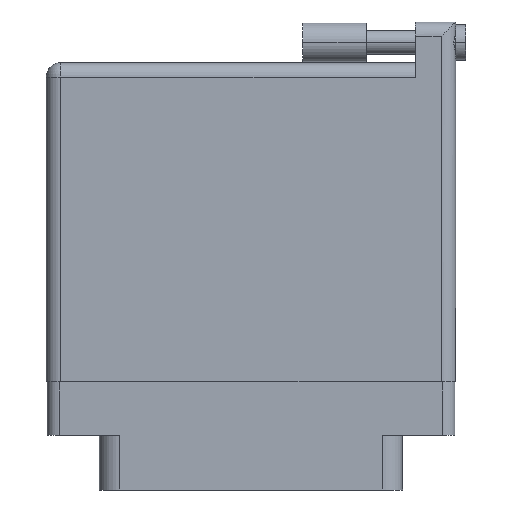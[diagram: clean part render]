
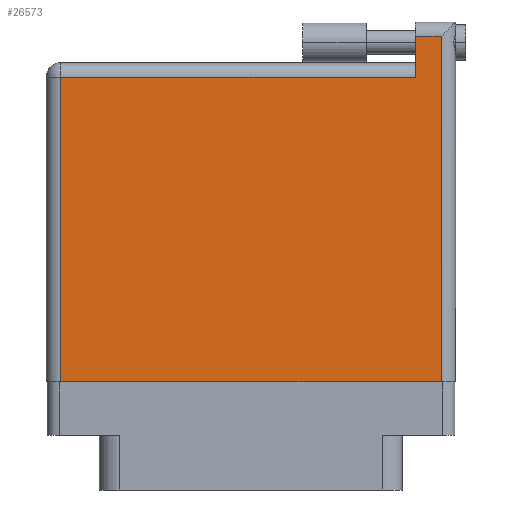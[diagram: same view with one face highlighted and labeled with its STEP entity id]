
A CAD part, front view. The second image highlights one B-rep face of the part: STEP entity #26573.
In plain terms, the highlighted face is planar.
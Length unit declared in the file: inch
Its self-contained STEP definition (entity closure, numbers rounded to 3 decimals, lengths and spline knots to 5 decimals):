
#132 = CARTESIAN_POINT ( 'NONE',  ( 1.938, 0., 0. ) ) ;
#151 = EDGE_CURVE ( 'NONE', #28569, #36948, #36484, .T. ) ;
#687 = LINE ( 'NONE', #1060, #37702 ) ;
#731 = EDGE_CURVE ( 'NONE', #36948, #12872, #7564, .T. ) ;
#1060 = CARTESIAN_POINT ( 'NONE',  ( 1.938, 1.766, 0. ) ) ;
#1543 = ORIENTED_EDGE ( 'NONE', *, *, #731, .T. ) ;
#2525 = EDGE_CURVE ( 'NONE', #10656, #7990, #35919, .T. ) ;
#2567 = DIRECTION ( 'NONE',  ( 1., 0., 0. ) ) ;
#6646 = EDGE_LOOP ( 'NONE', ( #20522, #17226, #30401, #1543, #36429, #10999 ) ) ;
#7318 = FACE_OUTER_BOUND ( 'NONE', #6646, .T. ) ;
#7564 = LINE ( 'NONE', #14222, #23853 ) ;
#7990 = VERTEX_POINT ( 'NONE', #132 ) ;
#8092 = EDGE_CURVE ( 'NONE', #7990, #28569, #687, .T. ) ;
#8253 = VERTEX_POINT ( 'NONE', #28527 ) ;
#10656 = VERTEX_POINT ( 'NONE', #20781 ) ;
#10724 = DIRECTION ( 'NONE',  ( 0., -1., 0. ) ) ;
#10999 = ORIENTED_EDGE ( 'NONE', *, *, #38059, .T. ) ;
#11106 = LINE ( 'NONE', #13863, #38313 ) ;
#12872 = VERTEX_POINT ( 'NONE', #20496 ) ;
#13474 = CARTESIAN_POINT ( 'NONE',  ( 0., 1.496, 0. ) ) ;
#13863 = CARTESIAN_POINT ( 'NONE',  ( 0.07, 0., 0. ) ) ;
#14222 = CARTESIAN_POINT ( 'NONE',  ( 1.811, 1.766, 0. ) ) ;
#14727 = DIRECTION ( 'NONE',  ( -1., 0., 0. ) ) ;
#17097 = VECTOR ( 'NONE', #2567, 39.37008 ) ;
#17226 = ORIENTED_EDGE ( 'NONE', *, *, #8092, .T. ) ;
#17677 = VECTOR ( 'NONE', #14727, 39.37008 ) ;
#18479 = CARTESIAN_POINT ( 'NONE',  ( 1.811, 1.696, 0. ) ) ;
#20496 = CARTESIAN_POINT ( 'NONE',  ( 1.811, 1.496, 0. ) ) ;
#20522 = ORIENTED_EDGE ( 'NONE', *, *, #2525, .T. ) ;
#20781 = CARTESIAN_POINT ( 'NONE',  ( 0.07, 0., 0. ) ) ;
#20800 = CARTESIAN_POINT ( 'NONE',  ( 0., 0., 0. ) ) ;
#21564 = CARTESIAN_POINT ( 'NONE',  ( 0., 1.696, 0. ) ) ;
#22882 = LINE ( 'NONE', #13474, #24484 ) ;
#22999 = PLANE ( 'NONE',  #26948 ) ;
#23853 = VECTOR ( 'NONE', #31707, 39.37008 ) ;
#24484 = VECTOR ( 'NONE', #28570, 39.37008 ) ;
#25181 = DIRECTION ( 'NONE',  ( 0., 0., -1. ) ) ;
#26573 = ADVANCED_FACE ( 'NONE', ( #7318 ), #22999, .F. ) ;
#26948 = AXIS2_PLACEMENT_3D ( 'NONE', #28512, #25181, #37933 ) ;
#27796 = CARTESIAN_POINT ( 'NONE',  ( 1.938, 1.696, 0. ) ) ;
#28512 = CARTESIAN_POINT ( 'NONE',  ( 0., 1.566, 0. ) ) ;
#28527 = CARTESIAN_POINT ( 'NONE',  ( 0.07, 1.496, 0. ) ) ;
#28569 = VERTEX_POINT ( 'NONE', #27796 ) ;
#28570 = DIRECTION ( 'NONE',  ( -1., 0., 0. ) ) ;
#30401 = ORIENTED_EDGE ( 'NONE', *, *, #151, .T. ) ;
#30508 = DIRECTION ( 'NONE',  ( 0., 1., 0. ) ) ;
#31707 = DIRECTION ( 'NONE',  ( 0., -1., 0. ) ) ;
#35919 = LINE ( 'NONE', #20800, #17097 ) ;
#36429 = ORIENTED_EDGE ( 'NONE', *, *, #38081, .T. ) ;
#36484 = LINE ( 'NONE', #21564, #17677 ) ;
#36948 = VERTEX_POINT ( 'NONE', #18479 ) ;
#37702 = VECTOR ( 'NONE', #30508, 39.37008 ) ;
#37933 = DIRECTION ( 'NONE',  ( -1., 0., 0. ) ) ;
#38059 = EDGE_CURVE ( 'NONE', #8253, #10656, #11106, .T. ) ;
#38081 = EDGE_CURVE ( 'NONE', #12872, #8253, #22882, .T. ) ;
#38313 = VECTOR ( 'NONE', #10724, 39.37008 ) ;
